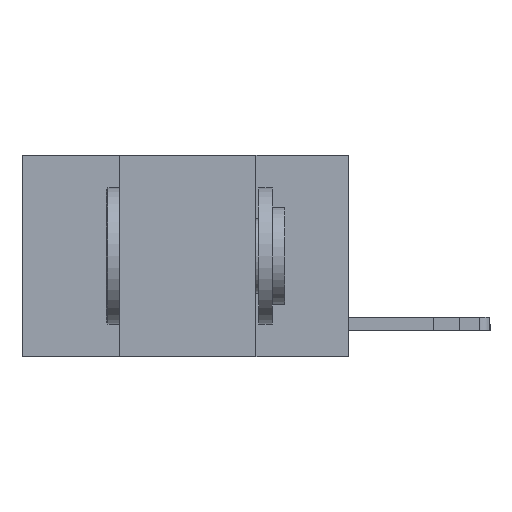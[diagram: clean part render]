
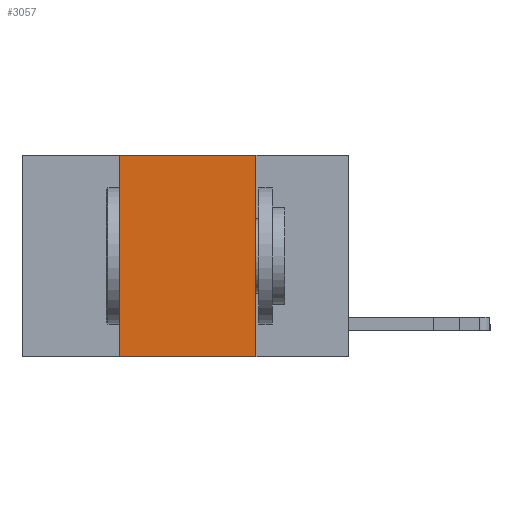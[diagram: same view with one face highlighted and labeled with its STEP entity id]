
A CAD part, left-side view. The second image highlights one B-rep face of the part: STEP entity #3057.
In plain terms, the highlighted planar face has unit normal (-1, 0, 0).
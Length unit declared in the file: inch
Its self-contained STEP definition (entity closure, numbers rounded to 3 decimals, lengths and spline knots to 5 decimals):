
#706 = LINE ( 'NONE', #19214, #4349 ) ;
#1114 = LINE ( 'NONE', #13452, #9375 ) ;
#1379 = EDGE_CURVE ( 'NONE', #16518, #14795, #17468, .T. ) ;
#1462 = CARTESIAN_POINT ( 'NONE',  ( 0., 0.17, 0. ) ) ;
#1779 = DIRECTION ( 'NONE',  ( 0., 0., -1. ) ) ;
#3057 = ADVANCED_FACE ( 'NONE', ( #15721 ), #17153, .F. ) ;
#3425 = DIRECTION ( 'NONE',  ( 0., -1., 0. ) ) ;
#3626 = CARTESIAN_POINT ( 'NONE',  ( 0., 0.6, 0. ) ) ;
#3975 = EDGE_CURVE ( 'NONE', #15267, #9117, #706, .T. ) ;
#4349 = VECTOR ( 'NONE', #13137, 39.37008 ) ;
#4566 = DIRECTION ( 'NONE',  ( 0., 0., 1. ) ) ;
#5501 = ORIENTED_EDGE ( 'NONE', *, *, #16759, .F. ) ;
#6611 = DIRECTION ( 'NONE',  ( 0., 0., -1. ) ) ;
#8710 = CARTESIAN_POINT ( 'NONE',  ( 0., 0.42, 0. ) ) ;
#8910 = CARTESIAN_POINT ( 'NONE',  ( 0., 0.42, -0.37 ) ) ;
#9117 = VERTEX_POINT ( 'NONE', #9437 ) ;
#9375 = VECTOR ( 'NONE', #4566, 39.37008 ) ;
#9437 = CARTESIAN_POINT ( 'NONE',  ( 0., 0.17, -0.37 ) ) ;
#9460 = CARTESIAN_POINT ( 'NONE',  ( 0., 0.6, 0. ) ) ;
#10548 = LINE ( 'NONE', #1462, #11164 ) ;
#10909 = EDGE_CURVE ( 'NONE', #14795, #9117, #10548, .T. ) ;
#11164 = VECTOR ( 'NONE', #6611, 39.37008 ) ;
#11929 = ORIENTED_EDGE ( 'NONE', *, *, #3975, .T. ) ;
#13137 = DIRECTION ( 'NONE',  ( 0., -1., 0. ) ) ;
#13452 = CARTESIAN_POINT ( 'NONE',  ( 0., 0.42, 0. ) ) ;
#14200 = VECTOR ( 'NONE', #3425, 39.37008 ) ;
#14795 = VERTEX_POINT ( 'NONE', #14893 ) ;
#14893 = CARTESIAN_POINT ( 'NONE',  ( 0., 0.17, 0. ) ) ;
#15267 = VERTEX_POINT ( 'NONE', #8910 ) ;
#15721 = FACE_OUTER_BOUND ( 'NONE', #16499, .T. ) ;
#15888 = ORIENTED_EDGE ( 'NONE', *, *, #1379, .F. ) ;
#16049 = AXIS2_PLACEMENT_3D ( 'NONE', #9460, #17345, #1779 ) ;
#16499 = EDGE_LOOP ( 'NONE', ( #18486, #15888, #5501, #11929 ) ) ;
#16518 = VERTEX_POINT ( 'NONE', #8710 ) ;
#16759 = EDGE_CURVE ( 'NONE', #15267, #16518, #1114, .T. ) ;
#17153 = PLANE ( 'NONE',  #16049 ) ;
#17345 = DIRECTION ( 'NONE',  ( 1., 0., 0. ) ) ;
#17468 = LINE ( 'NONE', #3626, #14200 ) ;
#18486 = ORIENTED_EDGE ( 'NONE', *, *, #10909, .F. ) ;
#19214 = CARTESIAN_POINT ( 'NONE',  ( 0., 0.6, -0.37 ) ) ;
